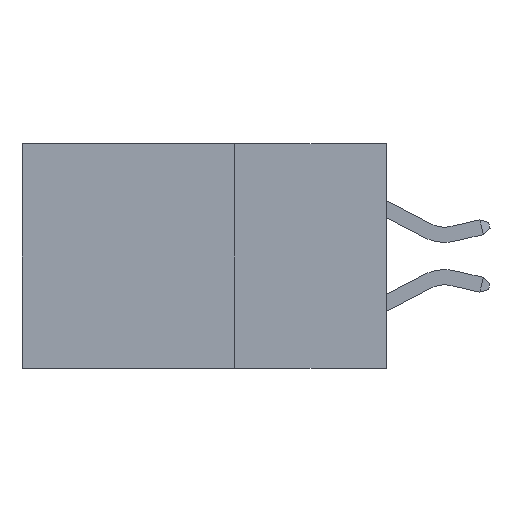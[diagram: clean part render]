
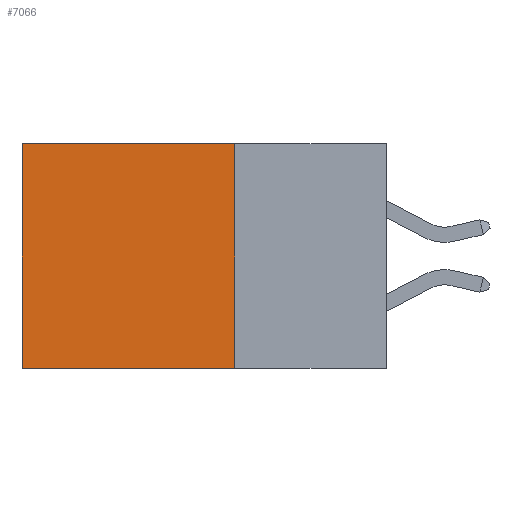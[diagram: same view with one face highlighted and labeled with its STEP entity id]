
A CAD part, left-side view. The second image highlights one B-rep face of the part: STEP entity #7066.
In plain terms, the highlighted planar face has unit normal (-1, 0, 0).
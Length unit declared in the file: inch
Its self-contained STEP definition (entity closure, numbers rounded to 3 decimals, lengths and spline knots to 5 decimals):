
#634 = AXIS2_PLACEMENT_3D ( 'NONE', #17936, #8782, #14859 ) ;
#807 = DIRECTION ( 'NONE',  ( 0., 0., -1. ) ) ;
#1307 = VERTEX_POINT ( 'NONE', #5130 ) ;
#2161 = CARTESIAN_POINT ( 'NONE',  ( 0.2615, 0.25, -0.37 ) ) ;
#2665 = ORIENTED_EDGE ( 'NONE', *, *, #12525, .T. ) ;
#2894 = PLANE ( 'NONE',  #634 ) ;
#2996 = FACE_OUTER_BOUND ( 'NONE', #18017, .T. ) ;
#3506 = CARTESIAN_POINT ( 'NONE',  ( 0.2615, 0.6, -0.37 ) ) ;
#4365 = DIRECTION ( 'NONE',  ( 0., 0., -1. ) ) ;
#4749 = CARTESIAN_POINT ( 'NONE',  ( 0.2615, 0.25, 0. ) ) ;
#5130 = CARTESIAN_POINT ( 'NONE',  ( 0.2615, 0.6, 0. ) ) ;
#5510 = VECTOR ( 'NONE', #807, 39.37008 ) ;
#6268 = EDGE_CURVE ( 'NONE', #1307, #13336, #12466, .T. ) ;
#7066 = ADVANCED_FACE ( 'NONE', ( #2996 ), #2894, .F. ) ;
#7727 = EDGE_CURVE ( 'NONE', #13331, #17779, #17302, .T. ) ;
#7747 = CARTESIAN_POINT ( 'NONE',  ( 0.2615, 0.6, -0.37 ) ) ;
#7939 = EDGE_CURVE ( 'NONE', #17779, #13336, #15174, .T. ) ;
#8077 = ORIENTED_EDGE ( 'NONE', *, *, #7939, .F. ) ;
#8782 = DIRECTION ( 'NONE',  ( 1., 0., 0. ) ) ;
#10057 = CARTESIAN_POINT ( 'NONE',  ( 0.2615, 0.25, -0.37 ) ) ;
#10647 = DIRECTION ( 'NONE',  ( 0., 1., 0. ) ) ;
#11880 = CARTESIAN_POINT ( 'NONE',  ( 0.2615, 0.25, -0.37 ) ) ;
#11949 = VECTOR ( 'NONE', #10647, 39.37008 ) ;
#12466 = LINE ( 'NONE', #3506, #5510 ) ;
#12525 = EDGE_CURVE ( 'NONE', #13331, #1307, #18767, .T. ) ;
#13022 = ORIENTED_EDGE ( 'NONE', *, *, #7727, .F. ) ;
#13064 = VECTOR ( 'NONE', #18663, 39.37008 ) ;
#13331 = VERTEX_POINT ( 'NONE', #4749 ) ;
#13336 = VERTEX_POINT ( 'NONE', #7747 ) ;
#14859 = DIRECTION ( 'NONE',  ( 0., 0., -1. ) ) ;
#15174 = LINE ( 'NONE', #11880, #11949 ) ;
#17302 = LINE ( 'NONE', #10057, #18090 ) ;
#17678 = ORIENTED_EDGE ( 'NONE', *, *, #6268, .T. ) ;
#17779 = VERTEX_POINT ( 'NONE', #2161 ) ;
#17936 = CARTESIAN_POINT ( 'NONE',  ( 0.2615, 0.25, -0.37 ) ) ;
#18017 = EDGE_LOOP ( 'NONE', ( #17678, #8077, #13022, #2665 ) ) ;
#18090 = VECTOR ( 'NONE', #4365, 39.37008 ) ;
#18379 = CARTESIAN_POINT ( 'NONE',  ( 0.2615, 0.25, 0. ) ) ;
#18663 = DIRECTION ( 'NONE',  ( 0., 1., 0. ) ) ;
#18767 = LINE ( 'NONE', #18379, #13064 ) ;
